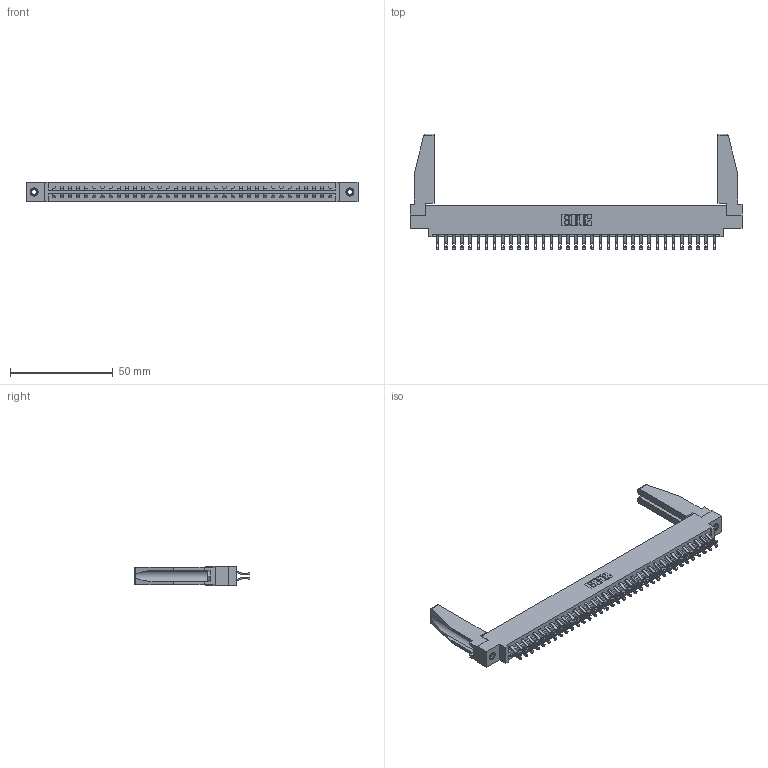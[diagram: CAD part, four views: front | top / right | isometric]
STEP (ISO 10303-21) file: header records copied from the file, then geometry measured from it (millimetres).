
FILE_DESCRIPTION (( 'STEP AP203' ), '1' );
FILE_NAME ('337-070-555-878.STEP', '2019-10-15T11:09:38', ( '' ), ( '' ), 'SwSTEP 2.0', 'SolidWorks 2016', '' );
FILE_SCHEMA (( 'CONFIG_CONTROL_DESIGN' ));
Length unit declared in the file: inch
Products named in the file (5): 307-220-078; 337 Part_0.170 Offset - 0.156 Dia-TI; 337-070-555-878; 345-250-001_345-250-001-102; 345-292-001_555 Tail
Assembly tree (75 placements, depth 2):
  337-070-555-878
    337 Part_0.170 Offset - 0.156 Dia-TI
    345-292-001_555 Tail  x70
    345-250-001_345-250-001-102  x2
    307-220-078  x2
Bounding box: 161.7 x 56.27 x 9.4 mm (x, y, z)
Volume: 21026.5 mm3; surface area: 23891.5 mm2
Topology: 75 solids, 75 shells, 4448 faces, 13883 edges, 9246 vertices
Faces by surface type: plane 2678, cylinder 1754, cone 12, torus 4
Entity records: 30940 total; most frequent: CARTESIAN_POINT 5254, ORIENTED_EDGE 5116, DIRECTION 4458, EDGE_CURVE 2558, VECTOR 2372, LINE 2372, VERTEX_POINT 1700, AXIS2_PLACEMENT_3D 1043
